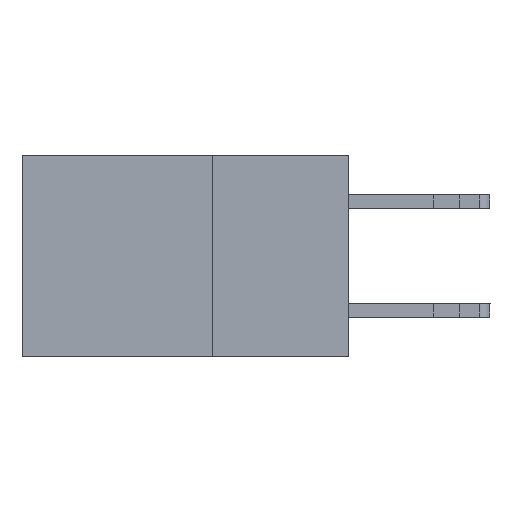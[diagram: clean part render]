
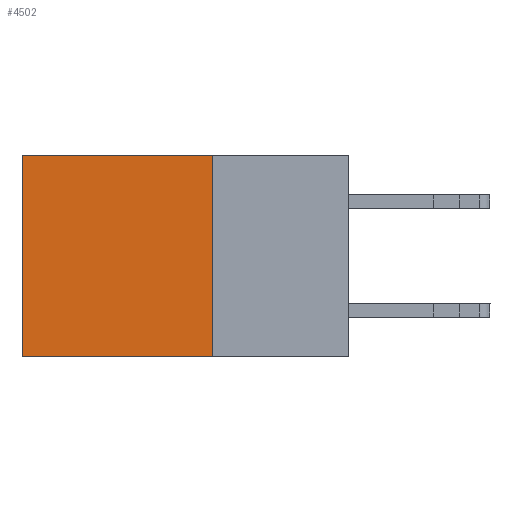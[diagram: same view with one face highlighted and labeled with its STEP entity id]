
A CAD part, left-side view. The second image highlights one B-rep face of the part: STEP entity #4502.
In plain terms, the highlighted planar face has unit normal (-1, 0, 0).
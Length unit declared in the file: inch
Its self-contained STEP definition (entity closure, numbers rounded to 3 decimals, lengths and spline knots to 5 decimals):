
#141 = DIRECTION ( 'NONE',  ( 0., 0., -1. ) ) ;
#201 = CARTESIAN_POINT ( 'NONE',  ( 0.2615, 0.25, -0.37 ) ) ;
#266 = CARTESIAN_POINT ( 'NONE',  ( 0.2615, 0.25, 0. ) ) ;
#748 = FACE_OUTER_BOUND ( 'NONE', #13887, .T. ) ;
#1543 = LINE ( 'NONE', #2415, #12454 ) ;
#1642 = ORIENTED_EDGE ( 'NONE', *, *, #14561, .F. ) ;
#1763 = DIRECTION ( 'NONE',  ( 0., 1., 0. ) ) ;
#2415 = CARTESIAN_POINT ( 'NONE',  ( 0.2615, 0.6, -0.37 ) ) ;
#2636 = LINE ( 'NONE', #15700, #13501 ) ;
#2672 = ORIENTED_EDGE ( 'NONE', *, *, #10312, .T. ) ;
#4464 = VERTEX_POINT ( 'NONE', #14657 ) ;
#4502 = ADVANCED_FACE ( 'NONE', ( #748 ), #13995, .F. ) ;
#4730 = VECTOR ( 'NONE', #1763, 39.37008 ) ;
#5185 = LINE ( 'NONE', #266, #4730 ) ;
#6817 = LINE ( 'NONE', #17068, #14287 ) ;
#7311 = DIRECTION ( 'NONE',  ( 0., 1., 0. ) ) ;
#7560 = AXIS2_PLACEMENT_3D ( 'NONE', #13945, #13684, #13649 ) ;
#9539 = DIRECTION ( 'NONE',  ( 0., 0., -1. ) ) ;
#9752 = ORIENTED_EDGE ( 'NONE', *, *, #11374, .T. ) ;
#10312 = EDGE_CURVE ( 'NONE', #17174, #4464, #5185, .T. ) ;
#11374 = EDGE_CURVE ( 'NONE', #4464, #14609, #1543, .T. ) ;
#12175 = EDGE_CURVE ( 'NONE', #14577, #14609, #2636, .T. ) ;
#12454 = VECTOR ( 'NONE', #9539, 39.37008 ) ;
#13501 = VECTOR ( 'NONE', #7311, 39.37008 ) ;
#13649 = DIRECTION ( 'NONE',  ( 0., 0., -1. ) ) ;
#13684 = DIRECTION ( 'NONE',  ( 1., 0., 0. ) ) ;
#13887 = EDGE_LOOP ( 'NONE', ( #9752, #18170, #1642, #2672 ) ) ;
#13945 = CARTESIAN_POINT ( 'NONE',  ( 0.2615, 0.25, -0.37 ) ) ;
#13995 = PLANE ( 'NONE',  #7560 ) ;
#14287 = VECTOR ( 'NONE', #141, 39.37008 ) ;
#14561 = EDGE_CURVE ( 'NONE', #17174, #14577, #6817, .T. ) ;
#14577 = VERTEX_POINT ( 'NONE', #201 ) ;
#14609 = VERTEX_POINT ( 'NONE', #17185 ) ;
#14657 = CARTESIAN_POINT ( 'NONE',  ( 0.2615, 0.6, 0. ) ) ;
#15498 = CARTESIAN_POINT ( 'NONE',  ( 0.2615, 0.25, 0. ) ) ;
#15700 = CARTESIAN_POINT ( 'NONE',  ( 0.2615, 0.25, -0.37 ) ) ;
#17068 = CARTESIAN_POINT ( 'NONE',  ( 0.2615, 0.25, -0.37 ) ) ;
#17174 = VERTEX_POINT ( 'NONE', #15498 ) ;
#17185 = CARTESIAN_POINT ( 'NONE',  ( 0.2615, 0.6, -0.37 ) ) ;
#18170 = ORIENTED_EDGE ( 'NONE', *, *, #12175, .F. ) ;
